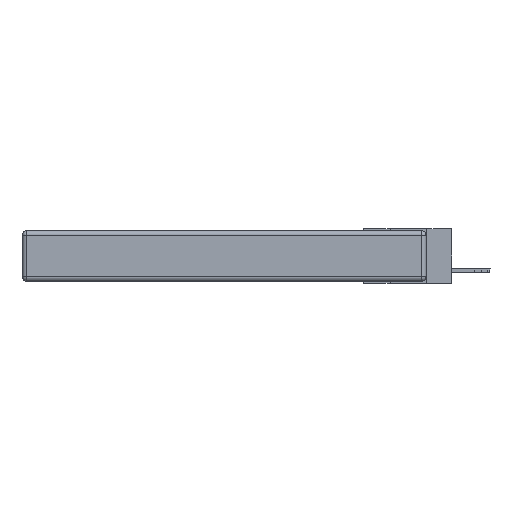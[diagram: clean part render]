
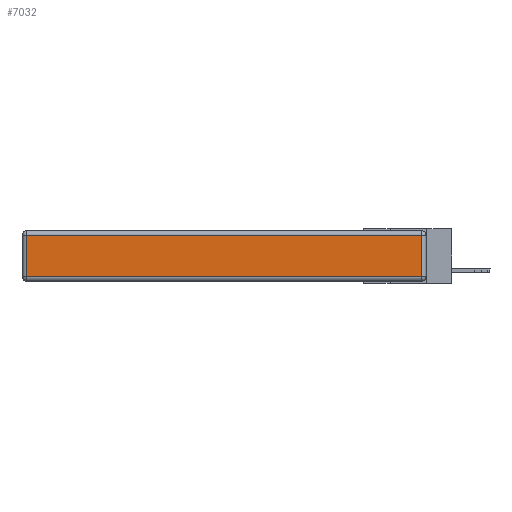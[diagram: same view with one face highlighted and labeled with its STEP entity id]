
A CAD part, left-side view. The second image highlights one B-rep face of the part: STEP entity #7032.
In plain terms, the highlighted planar face has unit normal (-1, 0, 0).
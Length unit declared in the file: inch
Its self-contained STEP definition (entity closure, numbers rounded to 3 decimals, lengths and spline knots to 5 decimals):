
#201 = EDGE_CURVE ( 'NONE', #7864, #2271, #15932, .T. ) ;
#225 = DIRECTION ( 'NONE',  ( 0., 0., 1. ) ) ;
#1225 = LINE ( 'NONE', #1562, #13311 ) ;
#1537 = VECTOR ( 'NONE', #17026, 39.37008 ) ;
#1562 = CARTESIAN_POINT ( 'NONE',  ( 0., 2.72, -0.343 ) ) ;
#2271 = VERTEX_POINT ( 'NONE', #12008 ) ;
#3865 = EDGE_LOOP ( 'NONE', ( #23014, #10818, #20233, #6268 ) ) ;
#4141 = CARTESIAN_POINT ( 'NONE',  ( 0., 0.03, -0.343 ) ) ;
#5206 = CARTESIAN_POINT ( 'NONE',  ( 0., 0., -0.313 ) ) ;
#5829 = PLANE ( 'NONE',  #7929 ) ;
#6268 = ORIENTED_EDGE ( 'NONE', *, *, #17366, .T. ) ;
#6446 = VERTEX_POINT ( 'NONE', #27476 ) ;
#6621 = FACE_OUTER_BOUND ( 'NONE', #3865, .T. ) ;
#7032 = ADVANCED_FACE ( 'NONE', ( #6621 ), #5829, .T. ) ;
#7076 = DIRECTION ( 'NONE',  ( 0., -1., 0. ) ) ;
#7864 = VERTEX_POINT ( 'NONE', #17776 ) ;
#7929 = AXIS2_PLACEMENT_3D ( 'NONE', #15374, #8955, #225 ) ;
#8955 = DIRECTION ( 'NONE',  ( -1., 0., 0. ) ) ;
#9152 = VECTOR ( 'NONE', #7076, 39.37008 ) ;
#9654 = CARTESIAN_POINT ( 'NONE',  ( 0., 0.03, -0.03 ) ) ;
#10178 = LINE ( 'NONE', #12759, #26675 ) ;
#10396 = DIRECTION ( 'NONE',  ( 0., 1., 0. ) ) ;
#10818 = ORIENTED_EDGE ( 'NONE', *, *, #17442, .T. ) ;
#12008 = CARTESIAN_POINT ( 'NONE',  ( 0., 0.03, -0.313 ) ) ;
#12759 = CARTESIAN_POINT ( 'NONE',  ( 0., 2.75, -0.03 ) ) ;
#12962 = LINE ( 'NONE', #4141, #1537 ) ;
#13311 = VECTOR ( 'NONE', #16655, 39.37008 ) ;
#15374 = CARTESIAN_POINT ( 'NONE',  ( 0., 0., -0.343 ) ) ;
#15932 = LINE ( 'NONE', #5206, #9152 ) ;
#16655 = DIRECTION ( 'NONE',  ( 0., 0., -1. ) ) ;
#17026 = DIRECTION ( 'NONE',  ( 0., 0., 1. ) ) ;
#17366 = EDGE_CURVE ( 'NONE', #6446, #7864, #1225, .T. ) ;
#17442 = EDGE_CURVE ( 'NONE', #2271, #23310, #12962, .T. ) ;
#17776 = CARTESIAN_POINT ( 'NONE',  ( 0., 2.72, -0.313 ) ) ;
#20233 = ORIENTED_EDGE ( 'NONE', *, *, #26254, .T. ) ;
#23014 = ORIENTED_EDGE ( 'NONE', *, *, #201, .T. ) ;
#23310 = VERTEX_POINT ( 'NONE', #9654 ) ;
#26254 = EDGE_CURVE ( 'NONE', #23310, #6446, #10178, .T. ) ;
#26675 = VECTOR ( 'NONE', #10396, 39.37008 ) ;
#27476 = CARTESIAN_POINT ( 'NONE',  ( 0., 2.72, -0.03 ) ) ;
